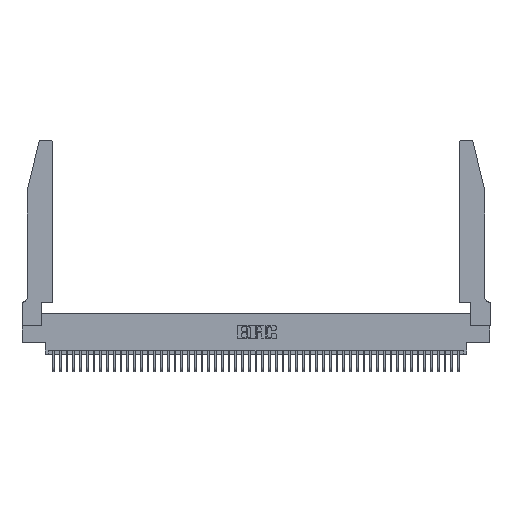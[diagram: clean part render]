
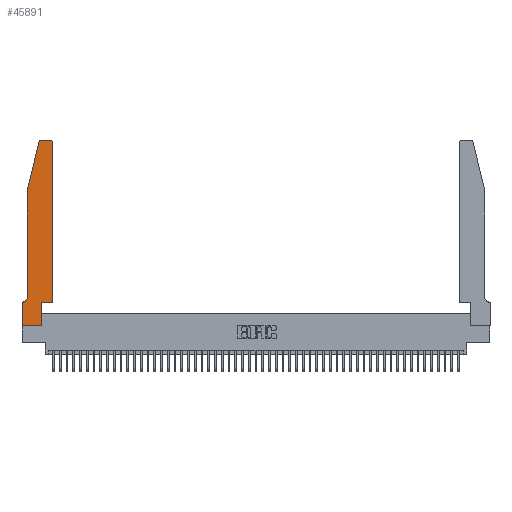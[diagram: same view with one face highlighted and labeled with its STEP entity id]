
A CAD part, top view. The second image highlights one B-rep face of the part: STEP entity #45891.
In plain terms, the highlighted planar face has unit normal (0, 0, 1).
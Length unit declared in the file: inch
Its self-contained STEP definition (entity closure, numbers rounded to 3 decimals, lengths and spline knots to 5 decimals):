
#23 = VERTEX_POINT ( 'NONE', #20225 ) ;
#374 = VECTOR ( 'NONE', #37633, 39.37008 ) ;
#1176 = VERTEX_POINT ( 'NONE', #43876 ) ;
#1765 = CARTESIAN_POINT ( 'NONE',  ( 0.284, 2.75, 0.37 ) ) ;
#2121 = VERTEX_POINT ( 'NONE', #10388 ) ;
#2200 = CARTESIAN_POINT ( 'NONE',  ( 0.0055, 0.42, 0.37 ) ) ;
#2457 = EDGE_CURVE ( 'NONE', #44566, #39109, #46022, .T. ) ;
#2572 = VECTOR ( 'NONE', #20428, 39.37008 ) ;
#2654 = VERTEX_POINT ( 'NONE', #17704 ) ;
#2895 = DIRECTION ( 'NONE',  ( 0., 0., 1. ) ) ;
#3407 = CARTESIAN_POINT ( 'NONE',  ( 0.0755, 0.35, 0.37 ) ) ;
#3541 = LINE ( 'NONE', #3407, #33055 ) ;
#4788 = CARTESIAN_POINT ( 'NONE',  ( 0., 0., 0.37 ) ) ;
#5477 = VERTEX_POINT ( 'NONE', #6742 ) ;
#5624 = DIRECTION ( 'NONE',  ( 0., 0., 1. ) ) ;
#5979 = CARTESIAN_POINT ( 'NONE',  ( 0.4505, 0.35, 0.37 ) ) ;
#6294 = DIRECTION ( 'NONE',  ( -1., 0., 0. ) ) ;
#6641 = CIRCLE ( 'NONE', #49724, 0.03 ) ;
#6742 = CARTESIAN_POINT ( 'NONE',  ( 0.2865, 0.35, 0.37 ) ) ;
#8777 = VECTOR ( 'NONE', #31145, 39.37008 ) ;
#9081 = EDGE_CURVE ( 'NONE', #2654, #23, #35780, .T. ) ;
#10359 = AXIS2_PLACEMENT_3D ( 'NONE', #26975, #2895, #30991 ) ;
#10388 = CARTESIAN_POINT ( 'NONE',  ( 0.4205, 2.75, 0.37 ) ) ;
#10712 = EDGE_CURVE ( 'NONE', #1176, #2654, #23290, .T. ) ;
#11397 = LINE ( 'NONE', #5979, #42071 ) ;
#11531 = DIRECTION ( 'NONE',  ( -1., 0., 0. ) ) ;
#11937 = EDGE_LOOP ( 'NONE', ( #13990, #51297, #22608, #35597, #29193, #34011, #48076, #36137, #24036, #46099, #22724, #35211 ) ) ;
#12338 = CARTESIAN_POINT ( 'NONE',  ( 0., 0.35, 0.37 ) ) ;
#12504 = AXIS2_PLACEMENT_3D ( 'NONE', #12338, #48360, #24433 ) ;
#12625 = CARTESIAN_POINT ( 'NONE',  ( 0.25487, 2.72718, 0.37 ) ) ;
#12836 = CARTESIAN_POINT ( 'NONE',  ( 0.4505, 0.35, 0.37 ) ) ;
#13434 = CARTESIAN_POINT ( 'NONE',  ( 0.0755, 2., 0.37 ) ) ;
#13666 = CARTESIAN_POINT ( 'NONE',  ( 0.0755, 2., 0.37 ) ) ;
#13990 = ORIENTED_EDGE ( 'NONE', *, *, #42811, .T. ) ;
#16366 = CARTESIAN_POINT ( 'NONE',  ( 0.0755, 2., 0.37 ) ) ;
#16961 = EDGE_CURVE ( 'NONE', #47518, #23453, #47592, .T. ) ;
#17704 = CARTESIAN_POINT ( 'NONE',  ( 0., 0., 0.37 ) ) ;
#18081 = CARTESIAN_POINT ( 'NONE',  ( 0., 0., 0.37 ) ) ;
#18871 = EDGE_CURVE ( 'NONE', #48347, #1176, #3541, .T. ) ;
#19998 = CARTESIAN_POINT ( 'NONE',  ( 0.2865, 0.35, 0.37 ) ) ;
#20225 = CARTESIAN_POINT ( 'NONE',  ( 0.2865, 0., 0.37 ) ) ;
#20428 = DIRECTION ( 'NONE',  ( -0.239, -0.971, 0. ) ) ;
#21820 = CIRCLE ( 'NONE', #49868, 0.07 ) ;
#22608 = ORIENTED_EDGE ( 'NONE', *, *, #38233, .T. ) ;
#22629 = CARTESIAN_POINT ( 'NONE',  ( 0.0055, 0.35, 0.37 ) ) ;
#22724 = ORIENTED_EDGE ( 'NONE', *, *, #2457, .T. ) ;
#22987 = EDGE_CURVE ( 'NONE', #5477, #44566, #11397, .T. ) ;
#23290 = LINE ( 'NONE', #18081, #42042 ) ;
#23453 = VERTEX_POINT ( 'NONE', #12625 ) ;
#24036 = ORIENTED_EDGE ( 'NONE', *, *, #48547, .T. ) ;
#24433 = DIRECTION ( 'NONE',  ( 1., 0., 0. ) ) ;
#25162 = VECTOR ( 'NONE', #36851, 39.37008 ) ;
#26488 = VERTEX_POINT ( 'NONE', #27297 ) ;
#26975 = CARTESIAN_POINT ( 'NONE',  ( 0.284, 2.72, 0.37 ) ) ;
#27297 = CARTESIAN_POINT ( 'NONE',  ( 0.0755, 0.42, 0.37 ) ) ;
#28291 = PLANE ( 'NONE',  #12504 ) ;
#29193 = ORIENTED_EDGE ( 'NONE', *, *, #40599, .T. ) ;
#29667 = CARTESIAN_POINT ( 'NONE',  ( 0.4205, 2.72, 0.37 ) ) ;
#30315 = DIRECTION ( 'NONE',  ( 0., 0., -1. ) ) ;
#30848 = LINE ( 'NONE', #16366, #2572 ) ;
#30991 = DIRECTION ( 'NONE',  ( 1., 0., 0. ) ) ;
#31145 = DIRECTION ( 'NONE',  ( 0., 1., 0. ) ) ;
#32551 = FACE_OUTER_BOUND ( 'NONE', #11937, .T. ) ;
#33055 = VECTOR ( 'NONE', #11531, 39.37008 ) ;
#33660 = CARTESIAN_POINT ( 'NONE',  ( 0.4505, 2.72, 0.37 ) ) ;
#33675 = DIRECTION ( 'NONE',  ( 1., 0., 0. ) ) ;
#34011 = ORIENTED_EDGE ( 'NONE', *, *, #18871, .T. ) ;
#34021 = DIRECTION ( 'NONE',  ( 1., 0., 0. ) ) ;
#34337 = VERTEX_POINT ( 'NONE', #13434 ) ;
#35001 = EDGE_CURVE ( 'NONE', #39109, #2121, #6641, .T. ) ;
#35104 = LINE ( 'NONE', #19998, #8777 ) ;
#35211 = ORIENTED_EDGE ( 'NONE', *, *, #35001, .T. ) ;
#35266 = LINE ( 'NONE', #37142, #44622 ) ;
#35394 = VECTOR ( 'NONE', #40813, 39.37008 ) ;
#35597 = ORIENTED_EDGE ( 'NONE', *, *, #46756, .T. ) ;
#35780 = LINE ( 'NONE', #4788, #25162 ) ;
#36137 = ORIENTED_EDGE ( 'NONE', *, *, #9081, .T. ) ;
#36851 = DIRECTION ( 'NONE',  ( 1., 0., 0. ) ) ;
#37142 = CARTESIAN_POINT ( 'NONE',  ( 0.2605, 2.75, 0.37 ) ) ;
#37633 = DIRECTION ( 'NONE',  ( 0., -1., 0. ) ) ;
#38233 = EDGE_CURVE ( 'NONE', #23453, #34337, #30848, .T. ) ;
#39109 = VERTEX_POINT ( 'NONE', #33660 ) ;
#40599 = EDGE_CURVE ( 'NONE', #26488, #48347, #21820, .T. ) ;
#40813 = DIRECTION ( 'NONE',  ( 0., 1., 0. ) ) ;
#42034 = DIRECTION ( 'NONE',  ( 0., -1., 0. ) ) ;
#42042 = VECTOR ( 'NONE', #42034, 39.37008 ) ;
#42071 = VECTOR ( 'NONE', #34021, 39.37008 ) ;
#42811 = EDGE_CURVE ( 'NONE', #2121, #47518, #35266, .T. ) ;
#43876 = CARTESIAN_POINT ( 'NONE',  ( 0., 0.35, 0.37 ) ) ;
#44143 = CARTESIAN_POINT ( 'NONE',  ( 0.4505, 0.35, 0.37 ) ) ;
#44566 = VERTEX_POINT ( 'NONE', #44143 ) ;
#44622 = VECTOR ( 'NONE', #45158, 39.37008 ) ;
#45158 = DIRECTION ( 'NONE',  ( -1., 0., 0. ) ) ;
#45543 = LINE ( 'NONE', #13666, #374 ) ;
#45891 = ADVANCED_FACE ( 'NONE', ( #32551 ), #28291, .T. ) ;
#46022 = LINE ( 'NONE', #12836, #35394 ) ;
#46099 = ORIENTED_EDGE ( 'NONE', *, *, #22987, .T. ) ;
#46756 = EDGE_CURVE ( 'NONE', #34337, #26488, #45543, .T. ) ;
#47518 = VERTEX_POINT ( 'NONE', #1765 ) ;
#47592 = CIRCLE ( 'NONE', #10359, 0.03 ) ;
#48076 = ORIENTED_EDGE ( 'NONE', *, *, #10712, .T. ) ;
#48347 = VERTEX_POINT ( 'NONE', #22629 ) ;
#48360 = DIRECTION ( 'NONE',  ( 0., 0., 1. ) ) ;
#48547 = EDGE_CURVE ( 'NONE', #23, #5477, #35104, .T. ) ;
#49724 = AXIS2_PLACEMENT_3D ( 'NONE', #29667, #5624, #33675 ) ;
#49868 = AXIS2_PLACEMENT_3D ( 'NONE', #2200, #30315, #6294 ) ;
#51297 = ORIENTED_EDGE ( 'NONE', *, *, #16961, .T. ) ;
